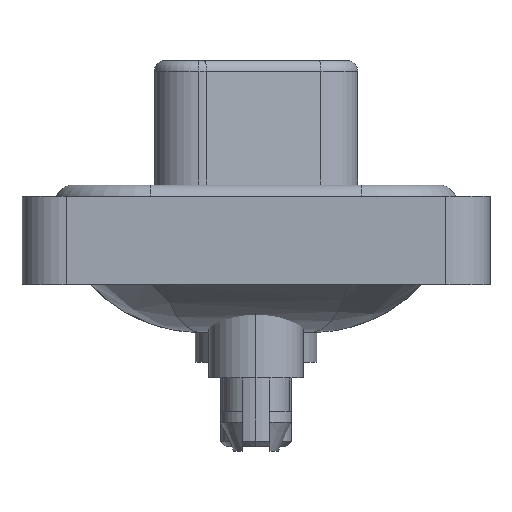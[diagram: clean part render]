
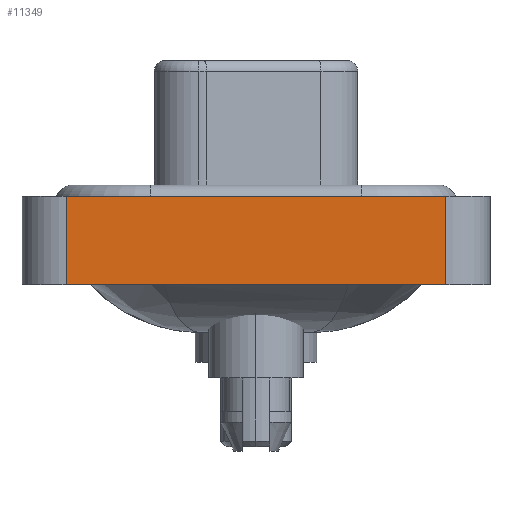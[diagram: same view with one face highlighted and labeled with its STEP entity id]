
A CAD part, left-side view. The second image highlights one B-rep face of the part: STEP entity #11349.
In plain terms, the highlighted planar face has unit normal (-1, 0, 0).
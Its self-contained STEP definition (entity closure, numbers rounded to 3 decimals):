
#385 = PLANE ( 'NONE',  #2761 ) ;
#600 = VECTOR ( 'NONE', #7711, 1000. ) ;
#783 = EDGE_CURVE ( 'NONE', #10267, #11265, #2701, .T. ) ;
#814 = LINE ( 'NONE', #8013, #10500 ) ;
#2701 = LINE ( 'NONE', #12833, #8544 ) ;
#2761 = AXIS2_PLACEMENT_3D ( 'NONE', #14375, #15585, #4023 ) ;
#2792 = LINE ( 'NONE', #6490, #600 ) ;
#3098 = CARTESIAN_POINT ( 'NONE',  ( -7.25, -8.55, -3.6 ) ) ;
#4023 = DIRECTION ( 'NONE',  ( 0., 0., 1. ) ) ;
#4181 = ORIENTED_EDGE ( 'NONE', *, *, #783, .F. ) ;
#4344 = EDGE_CURVE ( 'NONE', #11265, #10931, #10955, .T. ) ;
#5900 = VERTEX_POINT ( 'NONE', #3098 ) ;
#6490 = CARTESIAN_POINT ( 'NONE',  ( -7.25, -8.55, -3.6 ) ) ;
#7494 = EDGE_CURVE ( 'NONE', #10267, #5900, #2792, .T. ) ;
#7542 = ORIENTED_EDGE ( 'NONE', *, *, #7494, .T. ) ;
#7711 = DIRECTION ( 'NONE',  ( 0., -1., 0. ) ) ;
#8013 = CARTESIAN_POINT ( 'NONE',  ( -7.25, -8.55, -3.6 ) ) ;
#8066 = EDGE_LOOP ( 'NONE', ( #15616, #13323, #4181, #7542 ) ) ;
#8286 = VECTOR ( 'NONE', #13272, 1000. ) ;
#8432 = CARTESIAN_POINT ( 'NONE',  ( -7.25, 8.55, -3.6 ) ) ;
#8544 = VECTOR ( 'NONE', #13797, 1000. ) ;
#9667 = CARTESIAN_POINT ( 'NONE',  ( -7.25, -8.55, 0.4 ) ) ;
#10267 = VERTEX_POINT ( 'NONE', #8432 ) ;
#10500 = VECTOR ( 'NONE', #15483, 1000. ) ;
#10931 = VERTEX_POINT ( 'NONE', #13051 ) ;
#10955 = LINE ( 'NONE', #9667, #8286 ) ;
#11265 = VERTEX_POINT ( 'NONE', #14651 ) ;
#11349 = ADVANCED_FACE ( 'NONE', ( #12795 ), #385, .T. ) ;
#11738 = EDGE_CURVE ( 'NONE', #5900, #10931, #814, .T. ) ;
#12795 = FACE_OUTER_BOUND ( 'NONE', #8066, .T. ) ;
#12833 = CARTESIAN_POINT ( 'NONE',  ( -7.25, 8.55, -3.6 ) ) ;
#13051 = CARTESIAN_POINT ( 'NONE',  ( -7.25, -8.55, 0.4 ) ) ;
#13272 = DIRECTION ( 'NONE',  ( 0., -1., 0. ) ) ;
#13323 = ORIENTED_EDGE ( 'NONE', *, *, #4344, .F. ) ;
#13797 = DIRECTION ( 'NONE',  ( 0., 0., 1. ) ) ;
#14375 = CARTESIAN_POINT ( 'NONE',  ( -7.25, -8.55, -3.6 ) ) ;
#14651 = CARTESIAN_POINT ( 'NONE',  ( -7.25, 8.55, 0.4 ) ) ;
#15483 = DIRECTION ( 'NONE',  ( 0., 0., 1. ) ) ;
#15585 = DIRECTION ( 'NONE',  ( -1., 0., 0. ) ) ;
#15616 = ORIENTED_EDGE ( 'NONE', *, *, #11738, .T. ) ;
